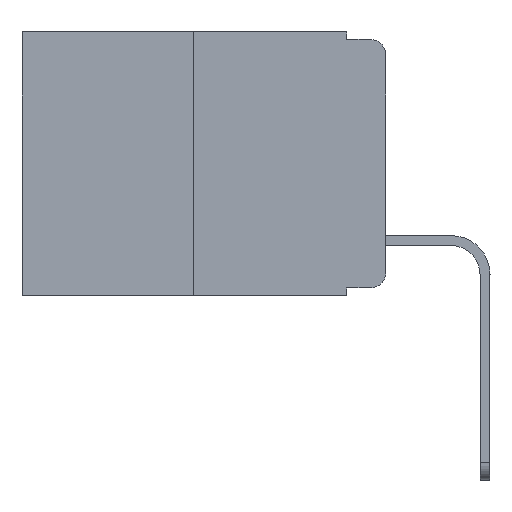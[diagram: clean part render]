
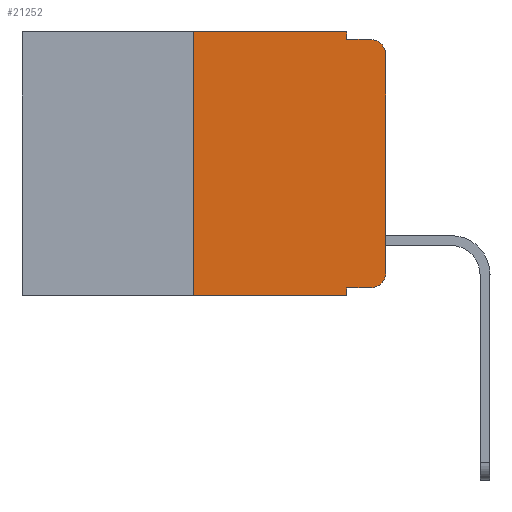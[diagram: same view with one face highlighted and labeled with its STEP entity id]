
A CAD part, left-side view. The second image highlights one B-rep face of the part: STEP entity #21252.
In plain terms, the highlighted planar face has unit normal (-1, 0, 0).
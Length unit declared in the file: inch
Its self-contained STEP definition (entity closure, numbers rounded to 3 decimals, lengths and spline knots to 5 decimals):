
#342 = DIRECTION ( 'NONE',  ( 0., 0., -1. ) ) ;
#507 = CARTESIAN_POINT ( 'NONE',  ( 0., 0.02, -0.333 ) ) ;
#1258 = DIRECTION ( 'NONE',  ( 0., 0., -1. ) ) ;
#1476 = CIRCLE ( 'NONE', #14561, 0.02 ) ;
#1532 = EDGE_LOOP ( 'NONE', ( #4022, #23143, #13777, #3382, #7145, #2877, #4812, #15470, #21695, #17851 ) ) ;
#1798 = DIRECTION ( 'NONE',  ( 0., -1., 0. ) ) ;
#2834 = EDGE_CURVE ( 'NONE', #18335, #7797, #10344, .T. ) ;
#2877 = ORIENTED_EDGE ( 'NONE', *, *, #8669, .F. ) ;
#3382 = ORIENTED_EDGE ( 'NONE', *, *, #21023, .F. ) ;
#4022 = ORIENTED_EDGE ( 'NONE', *, *, #18881, .T. ) ;
#4061 = VECTOR ( 'NONE', #7269, 39.37008 ) ;
#4072 = CARTESIAN_POINT ( 'NONE',  ( 0., 0.02, -0.01 ) ) ;
#4342 = EDGE_CURVE ( 'NONE', #7797, #19144, #14237, .T. ) ;
#4539 = VERTEX_POINT ( 'NONE', #9171 ) ;
#4622 = VERTEX_POINT ( 'NONE', #20872 ) ;
#4812 = ORIENTED_EDGE ( 'NONE', *, *, #5738, .T. ) ;
#5266 = VECTOR ( 'NONE', #9697, 39.37008 ) ;
#5282 = CARTESIAN_POINT ( 'NONE',  ( 0., 0.051, 0. ) ) ;
#5329 = CARTESIAN_POINT ( 'NONE',  ( 0., 0.02, -0.313 ) ) ;
#5359 = CARTESIAN_POINT ( 'NONE',  ( 0., 0.25, 0. ) ) ;
#5738 = EDGE_CURVE ( 'NONE', #8114, #12271, #9096, .T. ) ;
#5917 = CARTESIAN_POINT ( 'NONE',  ( 0., 0., -0.313 ) ) ;
#6246 = VECTOR ( 'NONE', #342, 39.37008 ) ;
#6337 = CARTESIAN_POINT ( 'NONE',  ( 0., 0.473, 0. ) ) ;
#6353 = LINE ( 'NONE', #5359, #4061 ) ;
#6639 = DIRECTION ( 'NONE',  ( 0., 0., 1. ) ) ;
#7145 = ORIENTED_EDGE ( 'NONE', *, *, #14810, .F. ) ;
#7269 = DIRECTION ( 'NONE',  ( 0., 0., 1. ) ) ;
#7770 = CARTESIAN_POINT ( 'NONE',  ( 0., 0.051, -0.343 ) ) ;
#7797 = VERTEX_POINT ( 'NONE', #507 ) ;
#8114 = VERTEX_POINT ( 'NONE', #8414 ) ;
#8414 = CARTESIAN_POINT ( 'NONE',  ( 0., 0.25, -0.343 ) ) ;
#8669 = EDGE_CURVE ( 'NONE', #8114, #16347, #6353, .T. ) ;
#8784 = VECTOR ( 'NONE', #1798, 39.37008 ) ;
#9016 = CARTESIAN_POINT ( 'NONE',  ( 0., 0.02, -0.03 ) ) ;
#9096 = LINE ( 'NONE', #20568, #16687 ) ;
#9106 = CARTESIAN_POINT ( 'NONE',  ( 0., 0.051, 0. ) ) ;
#9146 = VERTEX_POINT ( 'NONE', #4072 ) ;
#9171 = CARTESIAN_POINT ( 'NONE',  ( 0., 0.051, 0. ) ) ;
#9468 = VERTEX_POINT ( 'NONE', #18152 ) ;
#9697 = DIRECTION ( 'NONE',  ( 0., -1., 0. ) ) ;
#9883 = VECTOR ( 'NONE', #12221, 39.37008 ) ;
#10344 = LINE ( 'NONE', #18576, #5266 ) ;
#11076 = LINE ( 'NONE', #11974, #16137 ) ;
#11725 = EDGE_CURVE ( 'NONE', #18335, #12271, #15354, .T. ) ;
#11974 = CARTESIAN_POINT ( 'NONE',  ( 0., 0., 0. ) ) ;
#12221 = DIRECTION ( 'NONE',  ( 0., -1., 0. ) ) ;
#12271 = VERTEX_POINT ( 'NONE', #7770 ) ;
#12578 = EDGE_CURVE ( 'NONE', #4622, #9146, #1476, .T. ) ;
#12715 = LINE ( 'NONE', #5282, #6246 ) ;
#12786 = DIRECTION ( 'NONE',  ( -1., 0., 0. ) ) ;
#12972 = LINE ( 'NONE', #14514, #8784 ) ;
#13534 = LINE ( 'NONE', #6337, #9883 ) ;
#13777 = ORIENTED_EDGE ( 'NONE', *, *, #14473, .F. ) ;
#13809 = PLANE ( 'NONE',  #15897 ) ;
#13964 = CARTESIAN_POINT ( 'NONE',  ( 0., 0.051, -0.333 ) ) ;
#14237 = CIRCLE ( 'NONE', #16113, 0.02 ) ;
#14429 = DIRECTION ( 'NONE',  ( -1., 0., 0. ) ) ;
#14448 = DIRECTION ( 'NONE',  ( 0., 0., -1. ) ) ;
#14473 = EDGE_CURVE ( 'NONE', #9468, #9146, #12972, .T. ) ;
#14514 = CARTESIAN_POINT ( 'NONE',  ( 0., 0.051, -0.01 ) ) ;
#14561 = AXIS2_PLACEMENT_3D ( 'NONE', #9016, #14429, #21428 ) ;
#14810 = EDGE_CURVE ( 'NONE', #16347, #4539, #13534, .T. ) ;
#15354 = LINE ( 'NONE', #9106, #18450 ) ;
#15388 = DIRECTION ( 'NONE',  ( 1., 0., 0. ) ) ;
#15470 = ORIENTED_EDGE ( 'NONE', *, *, #11725, .F. ) ;
#15897 = AXIS2_PLACEMENT_3D ( 'NONE', #19013, #15388, #1258 ) ;
#16113 = AXIS2_PLACEMENT_3D ( 'NONE', #5329, #12786, #23320 ) ;
#16137 = VECTOR ( 'NONE', #6639, 39.37008 ) ;
#16347 = VERTEX_POINT ( 'NONE', #16658 ) ;
#16658 = CARTESIAN_POINT ( 'NONE',  ( 0., 0.25, 0. ) ) ;
#16687 = VECTOR ( 'NONE', #16944, 39.37008 ) ;
#16944 = DIRECTION ( 'NONE',  ( 0., -1., 0. ) ) ;
#17851 = ORIENTED_EDGE ( 'NONE', *, *, #4342, .T. ) ;
#18152 = CARTESIAN_POINT ( 'NONE',  ( 0., 0.051, -0.01 ) ) ;
#18335 = VERTEX_POINT ( 'NONE', #13964 ) ;
#18450 = VECTOR ( 'NONE', #14448, 39.37008 ) ;
#18576 = CARTESIAN_POINT ( 'NONE',  ( 0., 0.051, -0.333 ) ) ;
#18881 = EDGE_CURVE ( 'NONE', #19144, #4622, #11076, .T. ) ;
#18925 = FACE_OUTER_BOUND ( 'NONE', #1532, .T. ) ;
#19013 = CARTESIAN_POINT ( 'NONE',  ( 0., 0.473, 0. ) ) ;
#19144 = VERTEX_POINT ( 'NONE', #5917 ) ;
#20568 = CARTESIAN_POINT ( 'NONE',  ( 0., 0.473, -0.343 ) ) ;
#20872 = CARTESIAN_POINT ( 'NONE',  ( 0., 0., -0.03 ) ) ;
#21023 = EDGE_CURVE ( 'NONE', #4539, #9468, #12715, .T. ) ;
#21252 = ADVANCED_FACE ( 'NONE', ( #18925 ), #13809, .F. ) ;
#21428 = DIRECTION ( 'NONE',  ( 0., 0., -1. ) ) ;
#21695 = ORIENTED_EDGE ( 'NONE', *, *, #2834, .T. ) ;
#23143 = ORIENTED_EDGE ( 'NONE', *, *, #12578, .T. ) ;
#23320 = DIRECTION ( 'NONE',  ( 0., 0., -1. ) ) ;
